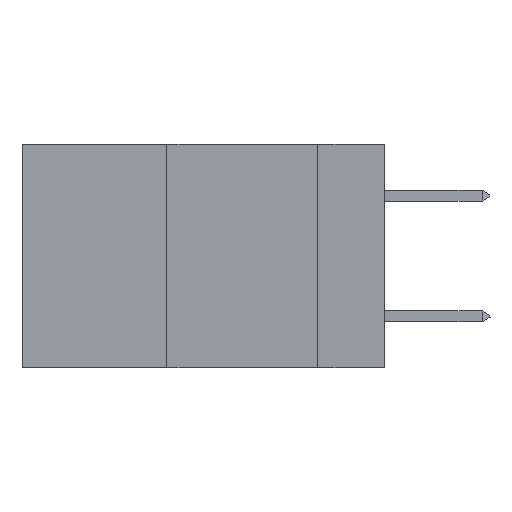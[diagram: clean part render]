
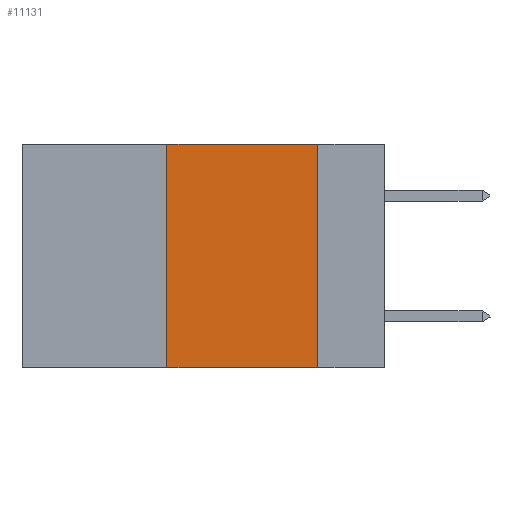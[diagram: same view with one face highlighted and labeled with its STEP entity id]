
A CAD part, left-side view. The second image highlights one B-rep face of the part: STEP entity #11131.
In plain terms, the highlighted planar face has unit normal (-1, 0, 0).
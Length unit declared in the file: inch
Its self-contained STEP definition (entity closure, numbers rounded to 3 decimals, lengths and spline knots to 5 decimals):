
#1728 = VECTOR ( 'NONE', #7916, 39.37008 ) ;
#1790 = ORIENTED_EDGE ( 'NONE', *, *, #7990, .F. ) ;
#2349 = VECTOR ( 'NONE', #13140, 39.37008 ) ;
#2654 = DIRECTION ( 'NONE',  ( 0., 0., -1. ) ) ;
#3101 = EDGE_CURVE ( 'NONE', #21639, #17615, #7072, .T. ) ;
#5642 = LINE ( 'NONE', #11351, #6218 ) ;
#5730 = CARTESIAN_POINT ( 'NONE',  ( 0., 0.36, 0. ) ) ;
#6218 = VECTOR ( 'NONE', #2654, 39.37008 ) ;
#7072 = LINE ( 'NONE', #20476, #2349 ) ;
#7916 = DIRECTION ( 'NONE',  ( 0., -1., 0. ) ) ;
#7990 = EDGE_CURVE ( 'NONE', #21127, #17615, #5642, .T. ) ;
#8415 = EDGE_LOOP ( 'NONE', ( #1790, #13352, #11599, #13052 ) ) ;
#8646 = EDGE_CURVE ( 'NONE', #8867, #21127, #11046, .T. ) ;
#8867 = VERTEX_POINT ( 'NONE', #11992 ) ;
#9270 = CARTESIAN_POINT ( 'NONE',  ( 0., 0.6, 0. ) ) ;
#10561 = CARTESIAN_POINT ( 'NONE',  ( 0., 0.11, -0.37 ) ) ;
#10957 = DIRECTION ( 'NONE',  ( 0., 0., -1. ) ) ;
#11046 = LINE ( 'NONE', #11333, #1728 ) ;
#11131 = ADVANCED_FACE ( 'NONE', ( #14212 ), #17700, .F. ) ;
#11234 = CARTESIAN_POINT ( 'NONE',  ( 0., 0.36, -0.37 ) ) ;
#11333 = CARTESIAN_POINT ( 'NONE',  ( 0., 0.6, 0. ) ) ;
#11351 = CARTESIAN_POINT ( 'NONE',  ( 0., 0.11, 0. ) ) ;
#11599 = ORIENTED_EDGE ( 'NONE', *, *, #20829, .F. ) ;
#11615 = CARTESIAN_POINT ( 'NONE',  ( 0., 0.11, 0. ) ) ;
#11992 = CARTESIAN_POINT ( 'NONE',  ( 0., 0.36, 0. ) ) ;
#13052 = ORIENTED_EDGE ( 'NONE', *, *, #3101, .T. ) ;
#13140 = DIRECTION ( 'NONE',  ( 0., -1., 0. ) ) ;
#13352 = ORIENTED_EDGE ( 'NONE', *, *, #8646, .F. ) ;
#14212 = FACE_OUTER_BOUND ( 'NONE', #8415, .T. ) ;
#15063 = AXIS2_PLACEMENT_3D ( 'NONE', #9270, #21023, #10957 ) ;
#17615 = VERTEX_POINT ( 'NONE', #10561 ) ;
#17700 = PLANE ( 'NONE',  #15063 ) ;
#18760 = VECTOR ( 'NONE', #19362, 39.37008 ) ;
#19275 = LINE ( 'NONE', #5730, #18760 ) ;
#19362 = DIRECTION ( 'NONE',  ( 0., 0., 1. ) ) ;
#20476 = CARTESIAN_POINT ( 'NONE',  ( 0., 0.6, -0.37 ) ) ;
#20829 = EDGE_CURVE ( 'NONE', #21639, #8867, #19275, .T. ) ;
#21023 = DIRECTION ( 'NONE',  ( 1., 0., 0. ) ) ;
#21127 = VERTEX_POINT ( 'NONE', #11615 ) ;
#21639 = VERTEX_POINT ( 'NONE', #11234 ) ;
